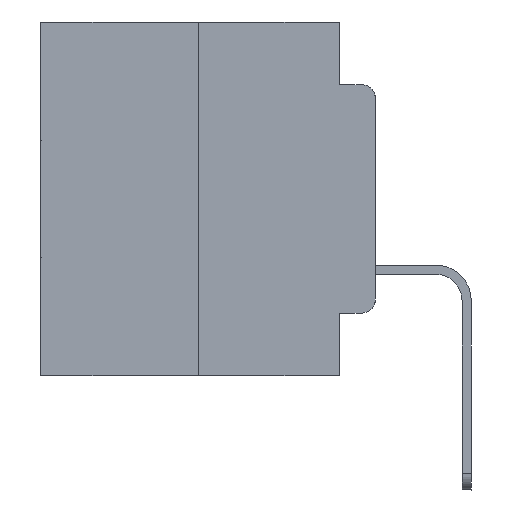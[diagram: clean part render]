
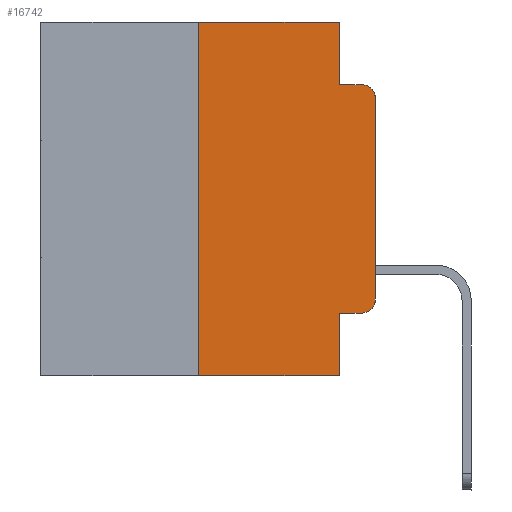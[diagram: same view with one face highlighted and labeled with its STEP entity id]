
A CAD part, left-side view. The second image highlights one B-rep face of the part: STEP entity #16742.
In plain terms, the highlighted planar face has unit normal (-1, 0, 0).
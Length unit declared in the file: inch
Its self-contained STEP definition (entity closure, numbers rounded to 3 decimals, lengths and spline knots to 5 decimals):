
#50 = LINE ( 'NONE', #17929, #21551 ) ;
#88 = DIRECTION ( 'NONE',  ( 0., 0., 1. ) ) ;
#423 = DIRECTION ( 'NONE',  ( 1., 0., 0. ) ) ;
#597 = VECTOR ( 'NONE', #9403, 39.37008 ) ;
#671 = CARTESIAN_POINT ( 'NONE',  ( 0., 0.051, -0.4115 ) ) ;
#681 = EDGE_CURVE ( 'NONE', #26317, #6024, #20812, .T. ) ;
#775 = CARTESIAN_POINT ( 'NONE',  ( 0., 0., -0.1085 ) ) ;
#976 = VECTOR ( 'NONE', #11346, 39.37008 ) ;
#1279 = CARTESIAN_POINT ( 'NONE',  ( 0., 0.02, -0.0885 ) ) ;
#2576 = CARTESIAN_POINT ( 'NONE',  ( 0., 0., 0. ) ) ;
#2582 = CARTESIAN_POINT ( 'NONE',  ( 0., 0.02, -0.3915 ) ) ;
#3154 = VECTOR ( 'NONE', #10511, 39.37008 ) ;
#3371 = ORIENTED_EDGE ( 'NONE', *, *, #681, .F. ) ;
#3653 = VERTEX_POINT ( 'NONE', #10745 ) ;
#3851 = DIRECTION ( 'NONE',  ( -1., 0., 0. ) ) ;
#4184 = CARTESIAN_POINT ( 'NONE',  ( 0., 0.051, 0. ) ) ;
#5422 = VERTEX_POINT ( 'NONE', #15263 ) ;
#6024 = VERTEX_POINT ( 'NONE', #13298 ) ;
#6182 = PLANE ( 'NONE',  #12153 ) ;
#6860 = ORIENTED_EDGE ( 'NONE', *, *, #24823, .F. ) ;
#7225 = LINE ( 'NONE', #671, #976 ) ;
#7233 = EDGE_CURVE ( 'NONE', #5422, #6024, #15652, .T. ) ;
#7246 = CARTESIAN_POINT ( 'NONE',  ( 0., 0.051, -0.4115 ) ) ;
#7770 = ORIENTED_EDGE ( 'NONE', *, *, #26960, .F. ) ;
#8227 = CARTESIAN_POINT ( 'NONE',  ( 0., 0.051, -0.0885 ) ) ;
#8427 = ORIENTED_EDGE ( 'NONE', *, *, #16807, .T. ) ;
#9271 = EDGE_CURVE ( 'NONE', #23906, #21580, #25989, .T. ) ;
#9403 = DIRECTION ( 'NONE',  ( 0., 0., -1. ) ) ;
#9516 = VERTEX_POINT ( 'NONE', #20961 ) ;
#10007 = CARTESIAN_POINT ( 'NONE',  ( 0., 0.25, 0. ) ) ;
#10156 = CARTESIAN_POINT ( 'NONE',  ( 0., 0.02, -0.1085 ) ) ;
#10511 = DIRECTION ( 'NONE',  ( 0., 0., -1. ) ) ;
#10745 = CARTESIAN_POINT ( 'NONE',  ( 0., 0., -0.3915 ) ) ;
#11346 = DIRECTION ( 'NONE',  ( 0., -1., 0. ) ) ;
#12153 = AXIS2_PLACEMENT_3D ( 'NONE', #26820, #423, #14447 ) ;
#12674 = AXIS2_PLACEMENT_3D ( 'NONE', #2582, #3851, #18449 ) ;
#13298 = CARTESIAN_POINT ( 'NONE',  ( 0., 0.051, -0.5 ) ) ;
#14447 = DIRECTION ( 'NONE',  ( 0., 0., -1. ) ) ;
#14758 = DIRECTION ( 'NONE',  ( 0., -1., 0. ) ) ;
#14860 = VERTEX_POINT ( 'NONE', #16191 ) ;
#15168 = EDGE_CURVE ( 'NONE', #26317, #14860, #7225, .T. ) ;
#15263 = CARTESIAN_POINT ( 'NONE',  ( 0., 0.25, -0.5 ) ) ;
#15339 = AXIS2_PLACEMENT_3D ( 'NONE', #10156, #24690, #16310 ) ;
#15652 = LINE ( 'NONE', #25216, #16948 ) ;
#15972 = LINE ( 'NONE', #2576, #26374 ) ;
#16191 = CARTESIAN_POINT ( 'NONE',  ( 0., 0.02, -0.4115 ) ) ;
#16310 = DIRECTION ( 'NONE',  ( 0., 0., -1. ) ) ;
#16742 = ADVANCED_FACE ( 'NONE', ( #25647 ), #6182, .F. ) ;
#16756 = ORIENTED_EDGE ( 'NONE', *, *, #15168, .T. ) ;
#16807 = EDGE_CURVE ( 'NONE', #14860, #3653, #23385, .T. ) ;
#16948 = VECTOR ( 'NONE', #14758, 39.37008 ) ;
#17039 = CARTESIAN_POINT ( 'NONE',  ( 0., 0.051, 0. ) ) ;
#17929 = CARTESIAN_POINT ( 'NONE',  ( 0., 0.473, 0. ) ) ;
#18020 = DIRECTION ( 'NONE',  ( 0., -1., 0. ) ) ;
#18427 = LINE ( 'NONE', #18897, #22006 ) ;
#18449 = DIRECTION ( 'NONE',  ( 0., 0., -1. ) ) ;
#18897 = CARTESIAN_POINT ( 'NONE',  ( 0., 0.25, 0. ) ) ;
#19754 = EDGE_CURVE ( 'NONE', #20630, #24036, #50, .T. ) ;
#19836 = LINE ( 'NONE', #8227, #26991 ) ;
#19992 = CARTESIAN_POINT ( 'NONE',  ( 0., 0.051, 0. ) ) ;
#20132 = EDGE_CURVE ( 'NONE', #3653, #23906, #15972, .T. ) ;
#20630 = VERTEX_POINT ( 'NONE', #10007 ) ;
#20812 = LINE ( 'NONE', #17039, #597 ) ;
#20842 = DIRECTION ( 'NONE',  ( 0., -1., 0. ) ) ;
#20907 = ORIENTED_EDGE ( 'NONE', *, *, #19754, .F. ) ;
#20961 = CARTESIAN_POINT ( 'NONE',  ( 0., 0.051, -0.0885 ) ) ;
#21551 = VECTOR ( 'NONE', #18020, 39.37008 ) ;
#21580 = VERTEX_POINT ( 'NONE', #1279 ) ;
#22006 = VECTOR ( 'NONE', #23091, 39.37008 ) ;
#22175 = ORIENTED_EDGE ( 'NONE', *, *, #25223, .F. ) ;
#23091 = DIRECTION ( 'NONE',  ( 0., 0., 1. ) ) ;
#23101 = ORIENTED_EDGE ( 'NONE', *, *, #7233, .T. ) ;
#23385 = CIRCLE ( 'NONE', #12674, 0.02 ) ;
#23906 = VERTEX_POINT ( 'NONE', #775 ) ;
#24023 = LINE ( 'NONE', #4184, #3154 ) ;
#24036 = VERTEX_POINT ( 'NONE', #19992 ) ;
#24611 = EDGE_LOOP ( 'NONE', ( #26545, #25518, #22175, #6860, #20907, #7770, #23101, #3371, #16756, #8427 ) ) ;
#24690 = DIRECTION ( 'NONE',  ( -1., 0., 0. ) ) ;
#24823 = EDGE_CURVE ( 'NONE', #24036, #9516, #24023, .T. ) ;
#25216 = CARTESIAN_POINT ( 'NONE',  ( 0., 0.473, -0.5 ) ) ;
#25223 = EDGE_CURVE ( 'NONE', #9516, #21580, #19836, .T. ) ;
#25518 = ORIENTED_EDGE ( 'NONE', *, *, #9271, .T. ) ;
#25647 = FACE_OUTER_BOUND ( 'NONE', #24611, .T. ) ;
#25989 = CIRCLE ( 'NONE', #15339, 0.02 ) ;
#26317 = VERTEX_POINT ( 'NONE', #7246 ) ;
#26374 = VECTOR ( 'NONE', #88, 39.37008 ) ;
#26545 = ORIENTED_EDGE ( 'NONE', *, *, #20132, .T. ) ;
#26820 = CARTESIAN_POINT ( 'NONE',  ( 0., 0.473, 0. ) ) ;
#26960 = EDGE_CURVE ( 'NONE', #5422, #20630, #18427, .T. ) ;
#26991 = VECTOR ( 'NONE', #20842, 39.37008 ) ;
